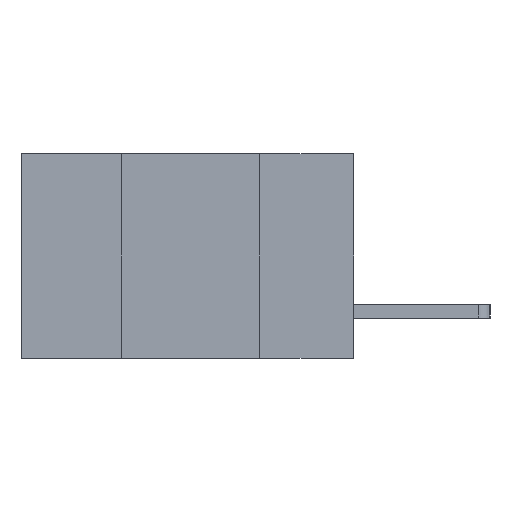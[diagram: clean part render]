
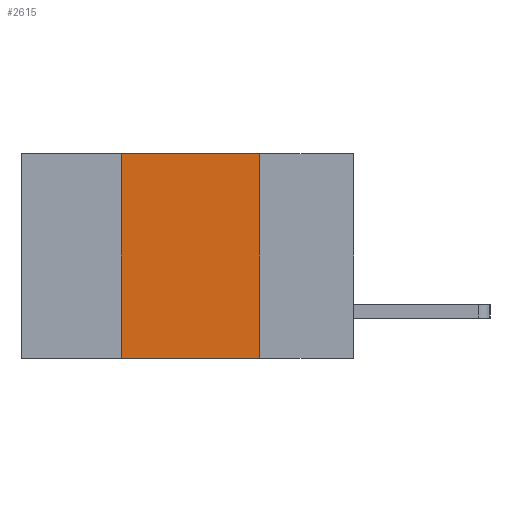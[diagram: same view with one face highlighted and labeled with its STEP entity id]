
A CAD part, left-side view. The second image highlights one B-rep face of the part: STEP entity #2615.
In plain terms, the highlighted planar face has unit normal (-1, 0, 0).
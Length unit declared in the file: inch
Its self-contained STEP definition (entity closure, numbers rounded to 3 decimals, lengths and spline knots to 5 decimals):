
#181 = ORIENTED_EDGE ( 'NONE', *, *, #9576, .F. ) ;
#686 = EDGE_CURVE ( 'NONE', #5021, #7521, #13544, .T. ) ;
#776 = VECTOR ( 'NONE', #10965, 39.37008 ) ;
#2615 = ADVANCED_FACE ( 'NONE', ( #7180 ), #5011, .F. ) ;
#2704 = CARTESIAN_POINT ( 'NONE',  ( 0., 0.17, 0. ) ) ;
#3381 = VERTEX_POINT ( 'NONE', #5458 ) ;
#3574 = VECTOR ( 'NONE', #12712, 39.37008 ) ;
#3600 = ORIENTED_EDGE ( 'NONE', *, *, #686, .T. ) ;
#4211 = LINE ( 'NONE', #9719, #776 ) ;
#5011 = PLANE ( 'NONE',  #9577 ) ;
#5021 = VERTEX_POINT ( 'NONE', #10075 ) ;
#5085 = DIRECTION ( 'NONE',  ( 1., 0., 0. ) ) ;
#5458 = CARTESIAN_POINT ( 'NONE',  ( 0., 0.42, 0. ) ) ;
#5739 = DIRECTION ( 'NONE',  ( 0., -1., 0. ) ) ;
#7180 = FACE_OUTER_BOUND ( 'NONE', #12225, .T. ) ;
#7521 = VERTEX_POINT ( 'NONE', #7544 ) ;
#7544 = CARTESIAN_POINT ( 'NONE',  ( 0., 0.17, -0.37 ) ) ;
#7670 = CARTESIAN_POINT ( 'NONE',  ( 0., 0.17, 0. ) ) ;
#8394 = CARTESIAN_POINT ( 'NONE',  ( 0., 0.6, 0. ) ) ;
#9129 = CARTESIAN_POINT ( 'NONE',  ( 0., 0.6, -0.37 ) ) ;
#9576 = EDGE_CURVE ( 'NONE', #5021, #3381, #4211, .T. ) ;
#9577 = AXIS2_PLACEMENT_3D ( 'NONE', #8394, #5085, #13842 ) ;
#9719 = CARTESIAN_POINT ( 'NONE',  ( 0., 0.42, 0. ) ) ;
#10037 = ORIENTED_EDGE ( 'NONE', *, *, #11276, .F. ) ;
#10075 = CARTESIAN_POINT ( 'NONE',  ( 0., 0.42, -0.37 ) ) ;
#10753 = LINE ( 'NONE', #14078, #11475 ) ;
#10965 = DIRECTION ( 'NONE',  ( 0., 0., 1. ) ) ;
#10967 = DIRECTION ( 'NONE',  ( 0., -1., 0. ) ) ;
#11276 = EDGE_CURVE ( 'NONE', #13332, #7521, #11629, .T. ) ;
#11372 = EDGE_CURVE ( 'NONE', #3381, #13332, #10753, .T. ) ;
#11475 = VECTOR ( 'NONE', #10967, 39.37008 ) ;
#11629 = LINE ( 'NONE', #2704, #3574 ) ;
#12225 = EDGE_LOOP ( 'NONE', ( #10037, #13569, #181, #3600 ) ) ;
#12712 = DIRECTION ( 'NONE',  ( 0., 0., -1. ) ) ;
#13332 = VERTEX_POINT ( 'NONE', #7670 ) ;
#13544 = LINE ( 'NONE', #9129, #13939 ) ;
#13569 = ORIENTED_EDGE ( 'NONE', *, *, #11372, .F. ) ;
#13842 = DIRECTION ( 'NONE',  ( 0., 0., -1. ) ) ;
#13939 = VECTOR ( 'NONE', #5739, 39.37008 ) ;
#14078 = CARTESIAN_POINT ( 'NONE',  ( 0., 0.6, 0. ) ) ;
